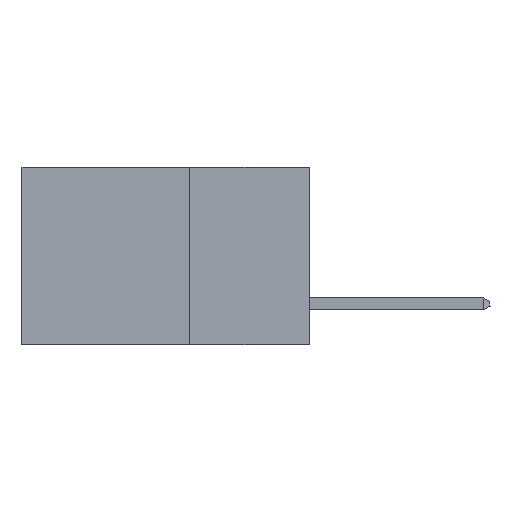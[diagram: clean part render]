
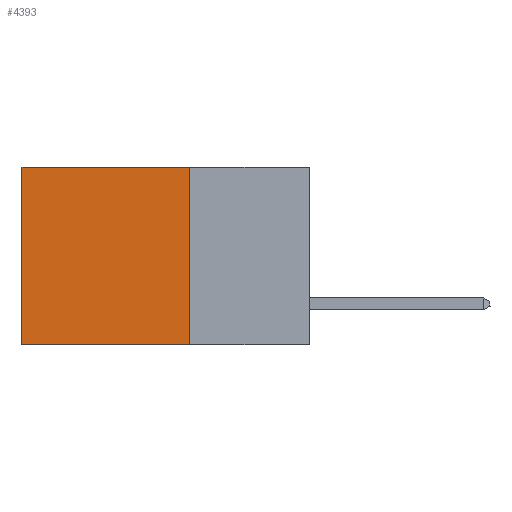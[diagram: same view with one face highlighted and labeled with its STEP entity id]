
A CAD part, left-side view. The second image highlights one B-rep face of the part: STEP entity #4393.
In plain terms, the highlighted planar face has unit normal (-1, 0, 0).
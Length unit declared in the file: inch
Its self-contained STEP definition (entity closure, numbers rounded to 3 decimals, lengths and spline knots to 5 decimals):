
#194 = CARTESIAN_POINT ( 'NONE',  ( 0.2875, 0.25, 0. ) ) ;
#1013 = VERTEX_POINT ( 'NONE', #11366 ) ;
#1129 = EDGE_CURVE ( 'NONE', #5853, #11649, #14096, .T. ) ;
#1322 = EDGE_CURVE ( 'NONE', #1013, #9430, #10574, .T. ) ;
#2736 = PLANE ( 'NONE',  #15721 ) ;
#3117 = CARTESIAN_POINT ( 'NONE',  ( 0.2875, 0.25, -0.37 ) ) ;
#3292 = EDGE_LOOP ( 'NONE', ( #12867, #11847, #7029, #7578 ) ) ;
#3547 = CARTESIAN_POINT ( 'NONE',  ( 0.2875, 0.25, 0. ) ) ;
#3990 = VECTOR ( 'NONE', #13920, 39.37008 ) ;
#4393 = ADVANCED_FACE ( 'NONE', ( #5629 ), #2736, .F. ) ;
#5281 = CARTESIAN_POINT ( 'NONE',  ( 0.2875, 0.6, 0. ) ) ;
#5629 = FACE_OUTER_BOUND ( 'NONE', #3292, .T. ) ;
#5853 = VERTEX_POINT ( 'NONE', #3547 ) ;
#6060 = CARTESIAN_POINT ( 'NONE',  ( 0.2875, 0.25, 0. ) ) ;
#7029 = ORIENTED_EDGE ( 'NONE', *, *, #7939, .F. ) ;
#7288 = VECTOR ( 'NONE', #13050, 39.37008 ) ;
#7578 = ORIENTED_EDGE ( 'NONE', *, *, #1129, .T. ) ;
#7939 = EDGE_CURVE ( 'NONE', #5853, #1013, #12200, .T. ) ;
#8324 = VECTOR ( 'NONE', #13639, 39.37008 ) ;
#9056 = DIRECTION ( 'NONE',  ( 0., 0., -1. ) ) ;
#9430 = VERTEX_POINT ( 'NONE', #12474 ) ;
#9573 = LINE ( 'NONE', #11090, #10937 ) ;
#10565 = EDGE_CURVE ( 'NONE', #11649, #9430, #9573, .T. ) ;
#10574 = LINE ( 'NONE', #3117, #7288 ) ;
#10937 = VECTOR ( 'NONE', #13812, 39.37008 ) ;
#11090 = CARTESIAN_POINT ( 'NONE',  ( 0.2875, 0.6, 0. ) ) ;
#11366 = CARTESIAN_POINT ( 'NONE',  ( 0.2875, 0.25, -0.37 ) ) ;
#11649 = VERTEX_POINT ( 'NONE', #5281 ) ;
#11847 = ORIENTED_EDGE ( 'NONE', *, *, #1322, .F. ) ;
#12200 = LINE ( 'NONE', #6060, #8324 ) ;
#12474 = CARTESIAN_POINT ( 'NONE',  ( 0.2875, 0.6, -0.37 ) ) ;
#12618 = DIRECTION ( 'NONE',  ( 1., 0., 0. ) ) ;
#12727 = CARTESIAN_POINT ( 'NONE',  ( 0.2875, 0.25, 0. ) ) ;
#12867 = ORIENTED_EDGE ( 'NONE', *, *, #10565, .T. ) ;
#13050 = DIRECTION ( 'NONE',  ( 0., 1., 0. ) ) ;
#13639 = DIRECTION ( 'NONE',  ( 0., 0., -1. ) ) ;
#13812 = DIRECTION ( 'NONE',  ( 0., 0., -1. ) ) ;
#13920 = DIRECTION ( 'NONE',  ( 0., 1., 0. ) ) ;
#14096 = LINE ( 'NONE', #194, #3990 ) ;
#15721 = AXIS2_PLACEMENT_3D ( 'NONE', #12727, #12618, #9056 ) ;
